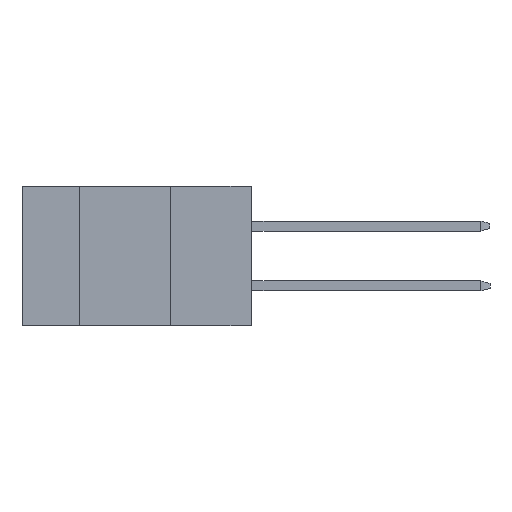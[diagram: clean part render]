
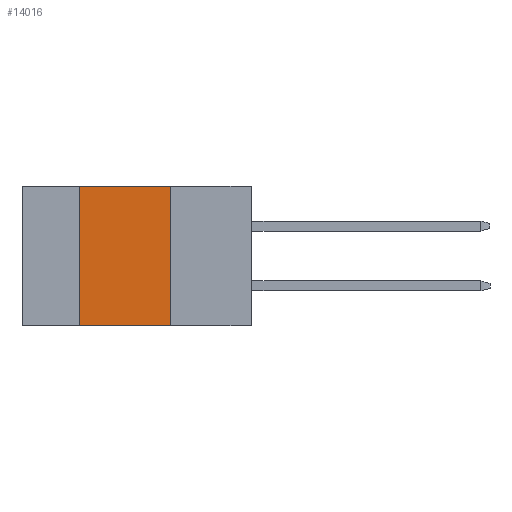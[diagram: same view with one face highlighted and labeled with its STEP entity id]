
A CAD part, left-side view. The second image highlights one B-rep face of the part: STEP entity #14016.
In plain terms, the highlighted planar face has unit normal (-1, 0, 0).
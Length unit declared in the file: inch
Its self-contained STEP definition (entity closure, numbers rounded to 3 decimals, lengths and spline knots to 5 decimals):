
#81 = LINE ( 'NONE', #12175, #11313 ) ;
#1541 = CARTESIAN_POINT ( 'NONE',  ( 0., 0.254, -0.437 ) ) ;
#2203 = CARTESIAN_POINT ( 'NONE',  ( 0., 0.254, -0.437 ) ) ;
#2311 = FACE_OUTER_BOUND ( 'NONE', #15192, .T. ) ;
#2813 = CARTESIAN_POINT ( 'NONE',  ( 0., 0.54, -0.437 ) ) ;
#2920 = ORIENTED_EDGE ( 'NONE', *, *, #3131, .F. ) ;
#3131 = EDGE_CURVE ( 'NONE', #14225, #10655, #12341, .T. ) ;
#3466 = VECTOR ( 'NONE', #9327, 39.37008 ) ;
#3632 = DIRECTION ( 'NONE',  ( 0., 0., -1. ) ) ;
#3668 = EDGE_CURVE ( 'NONE', #14225, #7165, #81, .T. ) ;
#4027 = EDGE_CURVE ( 'NONE', #15207, #7165, #10219, .T. ) ;
#4240 = DIRECTION ( 'NONE',  ( 0., -1., 0. ) ) ;
#6740 = VECTOR ( 'NONE', #8902, 39.37008 ) ;
#7165 = VERTEX_POINT ( 'NONE', #1541 ) ;
#7586 = ORIENTED_EDGE ( 'NONE', *, *, #8967, .F. ) ;
#7744 = CARTESIAN_POINT ( 'NONE',  ( 0., 0.72, 0. ) ) ;
#7812 = DIRECTION ( 'NONE',  ( 0., 0., -1. ) ) ;
#8045 = CARTESIAN_POINT ( 'NONE',  ( 0., 0.54, 0. ) ) ;
#8902 = DIRECTION ( 'NONE',  ( 0., -1., 0. ) ) ;
#8967 = EDGE_CURVE ( 'NONE', #10655, #15207, #12812, .T. ) ;
#9327 = DIRECTION ( 'NONE',  ( 0., 0., 1. ) ) ;
#9629 = VECTOR ( 'NONE', #7812, 39.37008 ) ;
#9936 = CARTESIAN_POINT ( 'NONE',  ( 0., 0.54, -0.437 ) ) ;
#10219 = LINE ( 'NONE', #2203, #9629 ) ;
#10655 = VERTEX_POINT ( 'NONE', #8045 ) ;
#11313 = VECTOR ( 'NONE', #4240, 39.37008 ) ;
#12130 = ORIENTED_EDGE ( 'NONE', *, *, #3668, .T. ) ;
#12175 = CARTESIAN_POINT ( 'NONE',  ( 0., 0.72, -0.437 ) ) ;
#12280 = AXIS2_PLACEMENT_3D ( 'NONE', #13765, #13670, #3632 ) ;
#12341 = LINE ( 'NONE', #2813, #3466 ) ;
#12812 = LINE ( 'NONE', #7744, #6740 ) ;
#13670 = DIRECTION ( 'NONE',  ( 1., 0., 0. ) ) ;
#13765 = CARTESIAN_POINT ( 'NONE',  ( 0., 0.72, 0. ) ) ;
#14016 = ADVANCED_FACE ( 'NONE', ( #2311 ), #17338, .F. ) ;
#14225 = VERTEX_POINT ( 'NONE', #9936 ) ;
#15192 = EDGE_LOOP ( 'NONE', ( #15978, #7586, #2920, #12130 ) ) ;
#15207 = VERTEX_POINT ( 'NONE', #16817 ) ;
#15978 = ORIENTED_EDGE ( 'NONE', *, *, #4027, .F. ) ;
#16817 = CARTESIAN_POINT ( 'NONE',  ( 0., 0.254, 0. ) ) ;
#17338 = PLANE ( 'NONE',  #12280 ) ;
